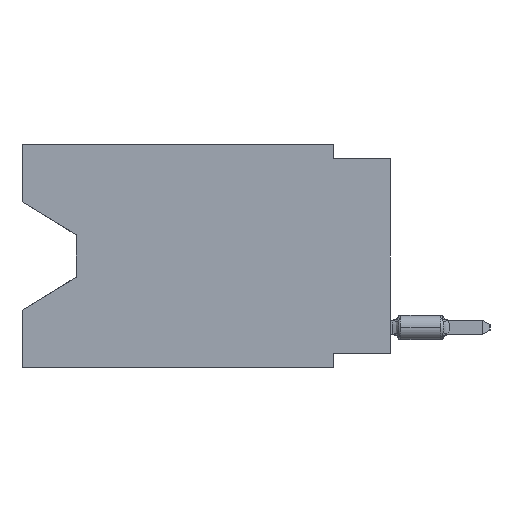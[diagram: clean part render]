
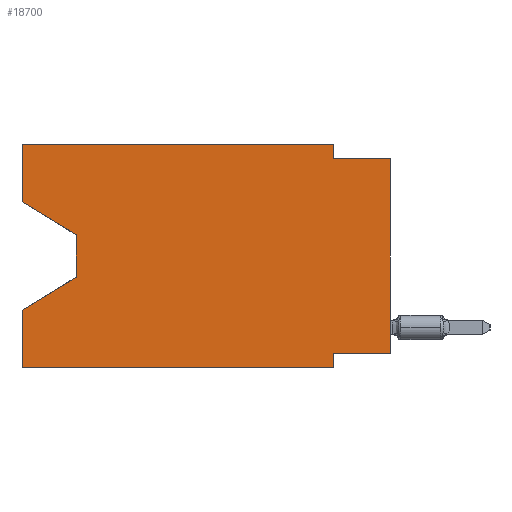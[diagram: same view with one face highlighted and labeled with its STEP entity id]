
A CAD part, left-side view. The second image highlights one B-rep face of the part: STEP entity #18700.
In plain terms, the highlighted planar face has unit normal (-1, 0, 0).
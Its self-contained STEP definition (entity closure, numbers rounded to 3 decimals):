
#51 = CARTESIAN_POINT ( 'NONE',  ( 0., 16.383, -9.906 ) ) ;
#582 = LINE ( 'NONE', #3564, #25672 ) ;
#875 = EDGE_CURVE ( 'NONE', #27965, #11426, #14133, .T. ) ;
#1410 = CARTESIAN_POINT ( 'NONE',  ( 0., 0., 0. ) ) ;
#2123 = EDGE_CURVE ( 'NONE', #6989, #8694, #33651, .T. ) ;
#2854 = LINE ( 'NONE', #4796, #28809 ) ;
#3124 = EDGE_CURVE ( 'NONE', #12711, #25770, #21129, .T. ) ;
#3564 = CARTESIAN_POINT ( 'NONE',  ( 0., 0., -0.635 ) ) ;
#3645 = VECTOR ( 'NONE', #22346, 1000. ) ;
#4036 = ORIENTED_EDGE ( 'NONE', *, *, #2123, .F. ) ;
#4796 = CARTESIAN_POINT ( 'NONE',  ( 0., 16.383, -2.546 ) ) ;
#5269 = VECTOR ( 'NONE', #29875, 1000. ) ;
#5273 = VECTOR ( 'NONE', #20340, 1000. ) ;
#5808 = CARTESIAN_POINT ( 'NONE',  ( 0., 0., -9.271 ) ) ;
#6470 = EDGE_LOOP ( 'NONE', ( #25833, #31770, #7682, #4036, #23420, #34604, #33501, #12443, #10087, #23688, #21181, #8050 ) ) ;
#6952 = LINE ( 'NONE', #17681, #21314 ) ;
#6971 = EDGE_CURVE ( 'NONE', #26233, #29888, #6952, .T. ) ;
#6989 = VERTEX_POINT ( 'NONE', #31006 ) ;
#7682 = ORIENTED_EDGE ( 'NONE', *, *, #10317, .T. ) ;
#8050 = ORIENTED_EDGE ( 'NONE', *, *, #875, .F. ) ;
#8236 = CARTESIAN_POINT ( 'NONE',  ( 0., 0., -0.635 ) ) ;
#8474 = AXIS2_PLACEMENT_3D ( 'NONE', #25710, #15519, #15340 ) ;
#8694 = VERTEX_POINT ( 'NONE', #28033 ) ;
#9617 = CARTESIAN_POINT ( 'NONE',  ( 0., 16.383, 0. ) ) ;
#9650 = CARTESIAN_POINT ( 'NONE',  ( 0., 16.383, 0. ) ) ;
#9697 = VECTOR ( 'NONE', #29418, 1000. ) ;
#9722 = VERTEX_POINT ( 'NONE', #23018 ) ;
#9976 = DIRECTION ( 'NONE',  ( 0., 0.855, -0.519 ) ) ;
#10087 = ORIENTED_EDGE ( 'NONE', *, *, #33743, .F. ) ;
#10310 = EDGE_CURVE ( 'NONE', #11426, #26233, #23318, .T. ) ;
#10317 = EDGE_CURVE ( 'NONE', #9722, #8694, #12601, .T. ) ;
#11426 = VERTEX_POINT ( 'NONE', #9650 ) ;
#12443 = ORIENTED_EDGE ( 'NONE', *, *, #28040, .T. ) ;
#12601 = LINE ( 'NONE', #34009, #32923 ) ;
#12711 = VERTEX_POINT ( 'NONE', #21423 ) ;
#13069 = DIRECTION ( 'NONE',  ( 0., -0.855, -0.519 ) ) ;
#13440 = LINE ( 'NONE', #51, #21223 ) ;
#13610 = DIRECTION ( 'NONE',  ( 0., -1., 0. ) ) ;
#14133 = LINE ( 'NONE', #34666, #9697 ) ;
#14144 = DIRECTION ( 'NONE',  ( 0., 0., -1. ) ) ;
#14195 = CARTESIAN_POINT ( 'NONE',  ( 0., 2.54, -0.635 ) ) ;
#14904 = CARTESIAN_POINT ( 'NONE',  ( 0., 16.383, 0. ) ) ;
#14992 = PLANE ( 'NONE',  #8474 ) ;
#15340 = DIRECTION ( 'NONE',  ( 0., 0., -1. ) ) ;
#15382 = VERTEX_POINT ( 'NONE', #8236 ) ;
#15519 = DIRECTION ( 'NONE',  ( 1., 0., 0. ) ) ;
#16617 = CARTESIAN_POINT ( 'NONE',  ( 0., 13.97, -4.013 ) ) ;
#16850 = VERTEX_POINT ( 'NONE', #34251 ) ;
#16947 = CARTESIAN_POINT ( 'NONE',  ( 0., 2.54, 0. ) ) ;
#17681 = CARTESIAN_POINT ( 'NONE',  ( 0., 2.54, 0. ) ) ;
#18700 = ADVANCED_FACE ( 'NONE', ( #25524 ), #14992, .F. ) ;
#19719 = LINE ( 'NONE', #27601, #3645 ) ;
#20234 = DIRECTION ( 'NONE',  ( 0., 0., 1. ) ) ;
#20340 = DIRECTION ( 'NONE',  ( 0., 0., 1. ) ) ;
#21129 = LINE ( 'NONE', #5808, #5269 ) ;
#21181 = ORIENTED_EDGE ( 'NONE', *, *, #10310, .F. ) ;
#21223 = VECTOR ( 'NONE', #13610, 1000. ) ;
#21314 = VECTOR ( 'NONE', #28046, 1000. ) ;
#21344 = VECTOR ( 'NONE', #14144, 1000. ) ;
#21423 = CARTESIAN_POINT ( 'NONE',  ( 0., 0., -9.271 ) ) ;
#22346 = DIRECTION ( 'NONE',  ( 0., 0., -1. ) ) ;
#22463 = EDGE_CURVE ( 'NONE', #27965, #28770, #2854, .T. ) ;
#23018 = CARTESIAN_POINT ( 'NONE',  ( 0., 13.97, -5.893 ) ) ;
#23318 = LINE ( 'NONE', #14904, #28450 ) ;
#23420 = ORIENTED_EDGE ( 'NONE', *, *, #30058, .T. ) ;
#23688 = ORIENTED_EDGE ( 'NONE', *, *, #6971, .F. ) ;
#23929 = VECTOR ( 'NONE', #20234, 1000. ) ;
#24283 = EDGE_CURVE ( 'NONE', #28770, #9722, #32222, .T. ) ;
#24305 = CARTESIAN_POINT ( 'NONE',  ( 0., 2.54, -9.271 ) ) ;
#25015 = DIRECTION ( 'NONE',  ( 0., -1., 0. ) ) ;
#25524 = FACE_OUTER_BOUND ( 'NONE', #6470, .T. ) ;
#25613 = DIRECTION ( 'NONE',  ( 0., -1., 0. ) ) ;
#25672 = VECTOR ( 'NONE', #25015, 1000. ) ;
#25677 = CARTESIAN_POINT ( 'NONE',  ( 0., 16.383, -2.546 ) ) ;
#25710 = CARTESIAN_POINT ( 'NONE',  ( 0., 16.383, 0. ) ) ;
#25770 = VERTEX_POINT ( 'NONE', #24305 ) ;
#25833 = ORIENTED_EDGE ( 'NONE', *, *, #22463, .T. ) ;
#26018 = LINE ( 'NONE', #1410, #23929 ) ;
#26233 = VERTEX_POINT ( 'NONE', #16947 ) ;
#26648 = EDGE_CURVE ( 'NONE', #25770, #16850, #19719, .T. ) ;
#27601 = CARTESIAN_POINT ( 'NONE',  ( 0., 2.54, -9.906 ) ) ;
#27703 = CARTESIAN_POINT ( 'NONE',  ( 0., 13.97, -4.013 ) ) ;
#27965 = VERTEX_POINT ( 'NONE', #25677 ) ;
#28033 = CARTESIAN_POINT ( 'NONE',  ( 0., 16.383, -7.36 ) ) ;
#28040 = EDGE_CURVE ( 'NONE', #12711, #15382, #26018, .T. ) ;
#28046 = DIRECTION ( 'NONE',  ( 0., 0., -1. ) ) ;
#28450 = VECTOR ( 'NONE', #25613, 1000. ) ;
#28770 = VERTEX_POINT ( 'NONE', #27703 ) ;
#28809 = VECTOR ( 'NONE', #13069, 1000. ) ;
#29418 = DIRECTION ( 'NONE',  ( 0., 0., 1. ) ) ;
#29875 = DIRECTION ( 'NONE',  ( 0., 1., 0. ) ) ;
#29888 = VERTEX_POINT ( 'NONE', #14195 ) ;
#30058 = EDGE_CURVE ( 'NONE', #6989, #16850, #13440, .T. ) ;
#31006 = CARTESIAN_POINT ( 'NONE',  ( 0., 16.383, -9.906 ) ) ;
#31770 = ORIENTED_EDGE ( 'NONE', *, *, #24283, .T. ) ;
#32222 = LINE ( 'NONE', #16617, #21344 ) ;
#32923 = VECTOR ( 'NONE', #9976, 1000. ) ;
#33501 = ORIENTED_EDGE ( 'NONE', *, *, #3124, .F. ) ;
#33651 = LINE ( 'NONE', #9617, #5273 ) ;
#33743 = EDGE_CURVE ( 'NONE', #29888, #15382, #582, .T. ) ;
#34009 = CARTESIAN_POINT ( 'NONE',  ( 0., 13.97, -5.893 ) ) ;
#34251 = CARTESIAN_POINT ( 'NONE',  ( 0., 2.54, -9.906 ) ) ;
#34604 = ORIENTED_EDGE ( 'NONE', *, *, #26648, .F. ) ;
#34666 = CARTESIAN_POINT ( 'NONE',  ( 0., 16.383, 0. ) ) ;
